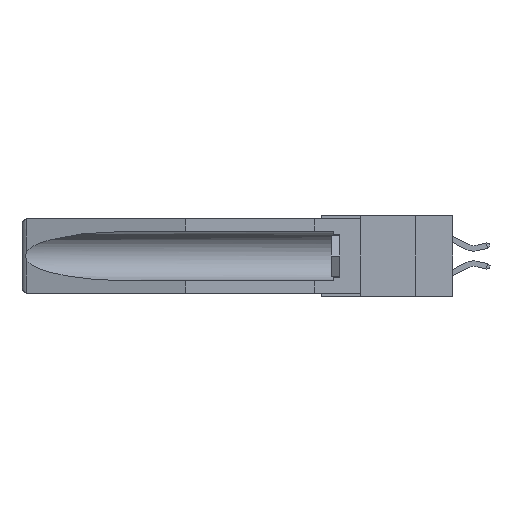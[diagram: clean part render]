
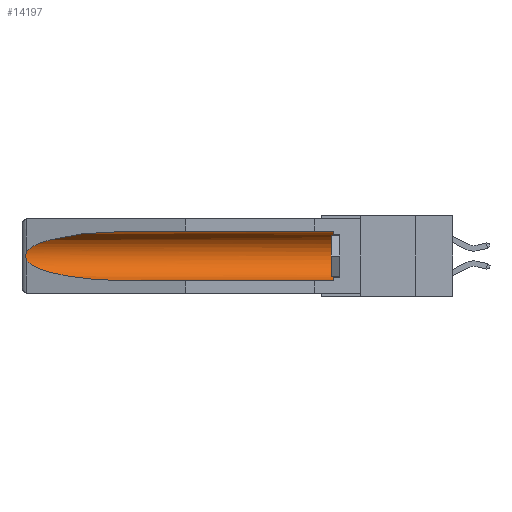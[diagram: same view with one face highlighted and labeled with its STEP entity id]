
A CAD part, left-side view. The second image highlights one B-rep face of the part: STEP entity #14197.
In plain terms, the highlighted cylindrical face has radius 2.857 mm (diameter 5.715 mm), a partial arc.
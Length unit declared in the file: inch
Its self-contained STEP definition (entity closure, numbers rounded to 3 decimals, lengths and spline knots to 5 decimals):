
#150 = CARTESIAN_POINT ( 'NONE',  ( 0.21114, 1.30732, -0.284 ) ) ;
#378 = ORIENTED_EDGE ( 'NONE', *, *, #12339, .F. ) ;
#896 = DIRECTION ( 'NONE',  ( 0., 0., 1. ) ) ;
#998 = AXIS2_PLACEMENT_3D ( 'NONE', #17385, #10055, #896 ) ;
#1156 = CARTESIAN_POINT ( 'NONE',  ( 0.26655, 1.53094, -0.18657 ) ) ;
#1167 = EDGE_CURVE ( 'NONE', #16926, #9918, #8267, .T. ) ;
#1539 = CARTESIAN_POINT ( 'NONE',  ( 0.26537, 1.52718, -0.19328 ) ) ;
#2213 = VERTEX_POINT ( 'NONE', #18910 ) ;
#2712 = CARTESIAN_POINT ( 'NONE',  ( 0.26597, 1.5296, -0.19026 ) ) ;
#4589 = CARTESIAN_POINT ( 'NONE',  ( 0.155, 1.07973, -0.284 ) ) ;
#4613 = CARTESIAN_POINT ( 'NONE',  ( 0.155, 1.07973, -0.284 ) ) ;
#4705 = CARTESIAN_POINT ( 'NONE',  ( 0.155, 0.126, -0.059 ) ) ;
#4814 = ORIENTED_EDGE ( 'NONE', *, *, #5328, .T. ) ;
#4828 = VECTOR ( 'NONE', #14524, 39.37008 ) ;
#5079 = DIRECTION ( 'NONE',  ( 0., 0., 1. ) ) ;
#5328 = EDGE_CURVE ( 'NONE', #2213, #16926, #10883, .T. ) ;
#5756 = EDGE_CURVE ( 'NONE', #12993, #8193, #18517, .T. ) ;
#5800 = CARTESIAN_POINT ( 'NONE',  ( 0.155, 0.126, -0.284 ) ) ;
#5864 = ORIENTED_EDGE ( 'NONE', *, *, #5756, .T. ) ;
#6042 = VERTEX_POINT ( 'NONE', #5800 ) ;
#6125 = EDGE_CURVE ( 'NONE', #8193, #2213, #19214, .T. ) ;
#6478 = CARTESIAN_POINT ( 'NONE',  ( 0.2675, 1.53308, -0.16763 ) ) ;
#6949 = CARTESIAN_POINT ( 'NONE',  ( 0.155, -0.30754, -0.059 ) ) ;
#7272 = ORIENTED_EDGE ( 'NONE', *, *, #1167, .T. ) ;
#7610 = CARTESIAN_POINT ( 'NONE',  ( 0.26537, 1.52718, -0.14972 ) ) ;
#7678 = CARTESIAN_POINT ( 'NONE',  ( 0.155, 1.07973, -0.059 ) ) ;
#8193 = VERTEX_POINT ( 'NONE', #17062 ) ;
#8267 =( BOUNDED_CURVE ( )  B_SPLINE_CURVE ( 3, ( #13525, #10533, #150, #4613 ),
 .UNSPECIFIED., .F., .F. ) 
 B_SPLINE_CURVE_WITH_KNOTS ( ( 4, 4 ),
 ( 0.1948, 1.5708 ),
 .UNSPECIFIED. ) 
 CURVE ( )  GEOMETRIC_REPRESENTATION_ITEM ( )  RATIONAL_B_SPLINE_CURVE ( ( 1., 0.848, 0.848, 1. ) ) 
 REPRESENTATION_ITEM ( '' )  );
#8770 = ORIENTED_EDGE ( 'NONE', *, *, #6125, .T. ) ;
#9148 = DIRECTION ( 'NONE',  ( 0., 1., 0. ) ) ;
#9918 = VERTEX_POINT ( 'NONE', #4589 ) ;
#9986 = CARTESIAN_POINT ( 'NONE',  ( 0.26537, 1.52718, -0.19328 ) ) ;
#10055 = DIRECTION ( 'NONE',  ( 0., -1., 0. ) ) ;
#10533 = CARTESIAN_POINT ( 'NONE',  ( 0.25451, 1.48313, -0.24835 ) ) ;
#10637 = ORIENTED_EDGE ( 'NONE', *, *, #17921, .T. ) ;
#10713 = FACE_OUTER_BOUND ( 'NONE', #15396, .T. ) ;
#10883 = B_SPLINE_CURVE_WITH_KNOTS ( 'NONE', 3,
 ( #12751, #15135, #16772, #18152, #6478, #18218, #12371, #1156, #2712, #9986 ),
 .UNSPECIFIED., .F., .F.,
 ( 4, 2, 2, 2, 4 ),
 ( 0., 0.00029, 0.00058, 0.00087, 0.00117 ),
 .UNSPECIFIED. ) ;
#12119 = CYLINDRICAL_SURFACE ( 'NONE', #12788, 0.1125 ) ;
#12142 = CARTESIAN_POINT ( 'NONE',  ( 0.155, -0.30754, -0.284 ) ) ;
#12159 = CARTESIAN_POINT ( 'NONE',  ( 0.25451, 1.48313, -0.09465 ) ) ;
#12339 = EDGE_CURVE ( 'NONE', #6042, #9918, #12694, .T. ) ;
#12371 = CARTESIAN_POINT ( 'NONE',  ( 0.2673, 1.53269, -0.17917 ) ) ;
#12506 = DIRECTION ( 'NONE',  ( 0., 1., 0. ) ) ;
#12694 = LINE ( 'NONE', #12142, #13618 ) ;
#12751 = CARTESIAN_POINT ( 'NONE',  ( 0.26537, 1.52718, -0.14972 ) ) ;
#12788 = AXIS2_PLACEMENT_3D ( 'NONE', #17157, #12506, #5079 ) ;
#12993 = VERTEX_POINT ( 'NONE', #4705 ) ;
#13525 = CARTESIAN_POINT ( 'NONE',  ( 0.26537, 1.52718, -0.19328 ) ) ;
#13618 = VECTOR ( 'NONE', #9148, 39.37008 ) ;
#14197 = ADVANCED_FACE ( 'NONE', ( #10713 ), #12119, .F. ) ;
#14524 = DIRECTION ( 'NONE',  ( 0., 1., 0. ) ) ;
#15135 = CARTESIAN_POINT ( 'NONE',  ( 0.26597, 1.52961, -0.15275 ) ) ;
#15396 = EDGE_LOOP ( 'NONE', ( #8770, #4814, #7272, #378, #10637, #5864 ) ) ;
#16500 = CARTESIAN_POINT ( 'NONE',  ( 0.21114, 1.30732, -0.059 ) ) ;
#16772 = CARTESIAN_POINT ( 'NONE',  ( 0.26654, 1.53092, -0.15636 ) ) ;
#16926 = VERTEX_POINT ( 'NONE', #1539 ) ;
#17062 = CARTESIAN_POINT ( 'NONE',  ( 0.155, 1.07973, -0.059 ) ) ;
#17157 = CARTESIAN_POINT ( 'NONE',  ( 0.155, -0.30754, -0.1715 ) ) ;
#17385 = CARTESIAN_POINT ( 'NONE',  ( 0.155, 0.126, -0.1715 ) ) ;
#17921 = EDGE_CURVE ( 'NONE', #6042, #12993, #18468, .T. ) ;
#18152 = CARTESIAN_POINT ( 'NONE',  ( 0.2673, 1.5327, -0.16383 ) ) ;
#18218 = CARTESIAN_POINT ( 'NONE',  ( 0.2675, 1.53308, -0.17534 ) ) ;
#18468 = CIRCLE ( 'NONE', #998, 0.1125 ) ;
#18517 = LINE ( 'NONE', #6949, #4828 ) ;
#18910 = CARTESIAN_POINT ( 'NONE',  ( 0.26537, 1.52718, -0.14972 ) ) ;
#19214 =( BOUNDED_CURVE ( )  B_SPLINE_CURVE ( 3, ( #7678, #16500, #12159, #7610 ),
 .UNSPECIFIED., .F., .F. ) 
 B_SPLINE_CURVE_WITH_KNOTS ( ( 4, 4 ),
 ( 4.71239, 6.08839 ),
 .UNSPECIFIED. ) 
 CURVE ( )  GEOMETRIC_REPRESENTATION_ITEM ( )  RATIONAL_B_SPLINE_CURVE ( ( 1., 0.848, 0.848, 1. ) ) 
 REPRESENTATION_ITEM ( '' )  );
